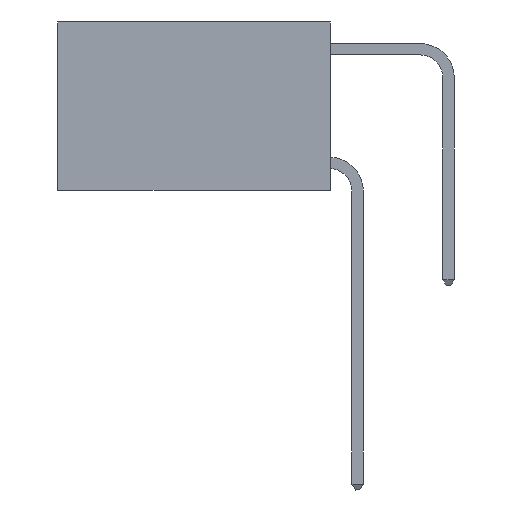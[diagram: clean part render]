
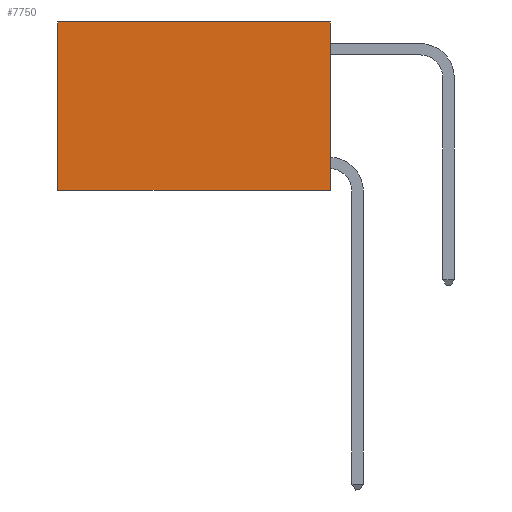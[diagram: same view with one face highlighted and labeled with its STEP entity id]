
A CAD part, left-side view. The second image highlights one B-rep face of the part: STEP entity #7750.
In plain terms, the highlighted planar face has unit normal (-1, 0, 0).
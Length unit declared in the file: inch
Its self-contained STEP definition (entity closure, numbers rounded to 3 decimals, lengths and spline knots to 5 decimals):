
#173 = VECTOR ( 'NONE', #10459, 39.37008 ) ;
#394 = VERTEX_POINT ( 'NONE', #6894 ) ;
#605 = DIRECTION ( 'NONE',  ( 0., 1., 0. ) ) ;
#800 = LINE ( 'NONE', #932, #11821 ) ;
#861 = CARTESIAN_POINT ( 'NONE',  ( 0.2625, 0.6, 0. ) ) ;
#932 = CARTESIAN_POINT ( 'NONE',  ( 0.2625, 0., 0. ) ) ;
#1377 = CARTESIAN_POINT ( 'NONE',  ( 0.2625, 0.6, 0. ) ) ;
#1491 = VECTOR ( 'NONE', #14998, 39.37008 ) ;
#1703 = LINE ( 'NONE', #15338, #173 ) ;
#2378 = DIRECTION ( 'NONE',  ( 0., 1., 0. ) ) ;
#2628 = VERTEX_POINT ( 'NONE', #5951 ) ;
#3185 = EDGE_CURVE ( 'NONE', #394, #14276, #7028, .T. ) ;
#3506 = ORIENTED_EDGE ( 'NONE', *, *, #6108, .F. ) ;
#3856 = PLANE ( 'NONE',  #14283 ) ;
#4546 = EDGE_CURVE ( 'NONE', #2628, #6384, #800, .T. ) ;
#5487 = VECTOR ( 'NONE', #605, 39.37008 ) ;
#5504 = ORIENTED_EDGE ( 'NONE', *, *, #4546, .T. ) ;
#5951 = CARTESIAN_POINT ( 'NONE',  ( 0.2625, 0., 0. ) ) ;
#6108 = EDGE_CURVE ( 'NONE', #2628, #394, #1703, .T. ) ;
#6179 = CARTESIAN_POINT ( 'NONE',  ( 0.2625, 0., 0. ) ) ;
#6384 = VERTEX_POINT ( 'NONE', #861 ) ;
#6864 = CARTESIAN_POINT ( 'NONE',  ( 0.2625, 0., -0.37 ) ) ;
#6894 = CARTESIAN_POINT ( 'NONE',  ( 0.2625, 0., -0.37 ) ) ;
#7015 = ORIENTED_EDGE ( 'NONE', *, *, #3185, .F. ) ;
#7028 = LINE ( 'NONE', #6864, #5487 ) ;
#7492 = LINE ( 'NONE', #1377, #1491 ) ;
#7750 = ADVANCED_FACE ( 'NONE', ( #11479 ), #3856, .F. ) ;
#8805 = DIRECTION ( 'NONE',  ( 0., 0., -1. ) ) ;
#8893 = ORIENTED_EDGE ( 'NONE', *, *, #14776, .T. ) ;
#9024 = CARTESIAN_POINT ( 'NONE',  ( 0.2625, 0.6, -0.37 ) ) ;
#10459 = DIRECTION ( 'NONE',  ( 0., 0., -1. ) ) ;
#11099 = DIRECTION ( 'NONE',  ( 1., 0., 0. ) ) ;
#11401 = EDGE_LOOP ( 'NONE', ( #8893, #7015, #3506, #5504 ) ) ;
#11479 = FACE_OUTER_BOUND ( 'NONE', #11401, .T. ) ;
#11821 = VECTOR ( 'NONE', #2378, 39.37008 ) ;
#14276 = VERTEX_POINT ( 'NONE', #9024 ) ;
#14283 = AXIS2_PLACEMENT_3D ( 'NONE', #6179, #11099, #8805 ) ;
#14776 = EDGE_CURVE ( 'NONE', #6384, #14276, #7492, .T. ) ;
#14998 = DIRECTION ( 'NONE',  ( 0., 0., -1. ) ) ;
#15338 = CARTESIAN_POINT ( 'NONE',  ( 0.2625, 0., 0. ) ) ;
